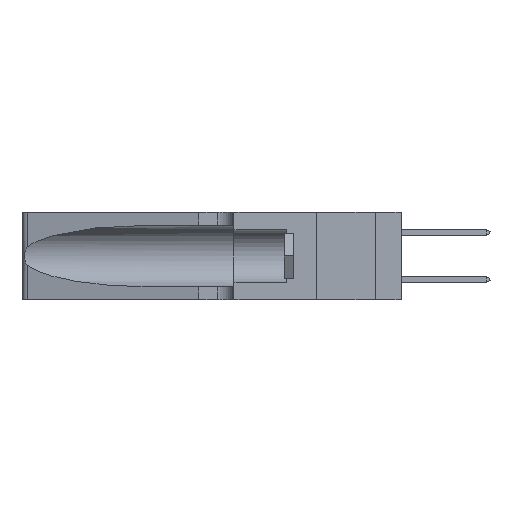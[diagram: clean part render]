
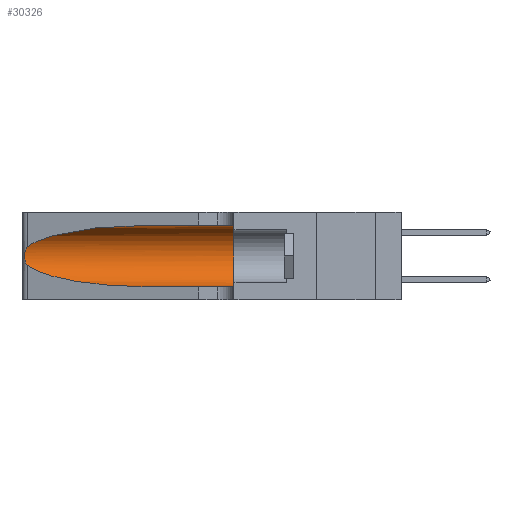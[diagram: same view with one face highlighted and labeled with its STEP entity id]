
A CAD part, left-side view. The second image highlights one B-rep face of the part: STEP entity #30326.
In plain terms, the highlighted cylindrical face has radius 3.308 mm (diameter 6.617 mm), a partial arc.
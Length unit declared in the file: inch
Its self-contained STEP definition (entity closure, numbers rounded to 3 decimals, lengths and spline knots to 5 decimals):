
#28 = ORIENTED_EDGE ( 'NONE', *, *, #17011, .T. ) ;
#201 = CARTESIAN_POINT ( 'NONE',  ( 0.25487, 1.22718, 0.22369 ) ) ;
#350 = CARTESIAN_POINT ( 'NONE',  ( 0.25639, 1.23186, 0.15144 ) ) ;
#483 = VECTOR ( 'NONE', #36586, 39.37008 ) ;
#2564 = AXIS2_PLACEMENT_3D ( 'NONE', #32352, #11757, #35770 ) ;
#2771 = CARTESIAN_POINT ( 'NONE',  ( 0.18966, 0.96281, 0.31525 ) ) ;
#3012 = CARTESIAN_POINT ( 'NONE',  ( 0.1305, 0.35, 0.31525 ) ) ;
#3841 = CARTESIAN_POINT ( 'NONE',  ( 0.25487, 1.22718, 0.14631 ) ) ;
#4213 = CARTESIAN_POINT ( 'NONE',  ( 0.2373, 1.15595, 0.08982 ) ) ;
#4339 = CARTESIAN_POINT ( 'NONE',  ( 0.1305, 0.35, 0.05475 ) ) ;
#5648 = CARTESIAN_POINT ( 'NONE',  ( 0.1305, 1.61858, 0.31525 ) ) ;
#6294 = CARTESIAN_POINT ( 'NONE',  ( 0.2373, 1.15595, 0.28018 ) ) ;
#7116 = VERTEX_POINT ( 'NONE', #38275 ) ;
#7188 = CARTESIAN_POINT ( 'NONE',  ( 0.25639, 1.23184, 0.21858 ) ) ;
#8153 = ORIENTED_EDGE ( 'NONE', *, *, #41227, .T. ) ;
#9260 = DIRECTION ( 'NONE',  ( 0., 0., -1. ) ) ;
#9715 = LINE ( 'NONE', #5648, #483 ) ;
#10643 = CARTESIAN_POINT ( 'NONE',  ( 0.25854, 1.2359, 0.20912 ) ) ;
#11147 = CARTESIAN_POINT ( 'NONE',  ( 0.1305, 0.72297, 0.05475 ) ) ;
#11757 = DIRECTION ( 'NONE',  ( 0., 1., 0. ) ) ;
#12356 = VERTEX_POINT ( 'NONE', #4339 ) ;
#14110 = CARTESIAN_POINT ( 'NONE',  ( 0.26075, 1.23896, 0.19203 ) ) ;
#14637 = ORIENTED_EDGE ( 'NONE', *, *, #16040, .F. ) ;
#16040 = EDGE_CURVE ( 'NONE', #32694, #33945, #9715, .T. ) ;
#16233 = VECTOR ( 'NONE', #33271, 39.37008 ) ;
#16890 = CIRCLE ( 'NONE', #2564, 0.13025 ) ;
#17011 = EDGE_CURVE ( 'NONE', #7116, #24454, #36749, .T. ) ;
#17569 = CARTESIAN_POINT ( 'NONE',  ( 0.26017, 1.23833, 0.17102 ) ) ;
#18398 = ORIENTED_EDGE ( 'NONE', *, *, #20824, .T. ) ;
#20617 = CYLINDRICAL_SURFACE ( 'NONE', #24099, 0.13025 ) ;
#20822 =( BOUNDED_CURVE ( )  B_SPLINE_CURVE ( 3, ( #28304, #4213, #31745, #11147 ),
 .UNSPECIFIED., .F., .F. ) 
 B_SPLINE_CURVE_WITH_KNOTS ( ( 4, 4 ),
 ( 3.44316, 4.71239 ),
 .UNSPECIFIED. ) 
 CURVE ( )  GEOMETRIC_REPRESENTATION_ITEM ( )  RATIONAL_B_SPLINE_CURVE ( ( 1., 0.87, 0.87, 1. ) ) 
 REPRESENTATION_ITEM ( '' )  );
#20824 = EDGE_CURVE ( 'NONE', #24454, #41369, #20822, .T. ) ;
#20894 = CARTESIAN_POINT ( 'NONE',  ( 0.25555, 1.22994, 0.2215 ) ) ;
#21042 = CARTESIAN_POINT ( 'NONE',  ( 0.25789, 1.23486, 0.15765 ) ) ;
#21650 = ORIENTED_EDGE ( 'NONE', *, *, #35269, .F. ) ;
#22866 = CARTESIAN_POINT ( 'NONE',  ( 0.25487, 1.22718, 0.14631 ) ) ;
#22958 = CARTESIAN_POINT ( 'NONE',  ( 0.1305, 1.61858, 0.185 ) ) ;
#24099 = AXIS2_PLACEMENT_3D ( 'NONE', #22958, #29871, #9260 ) ;
#24454 = VERTEX_POINT ( 'NONE', #22866 ) ;
#24498 = CARTESIAN_POINT ( 'NONE',  ( 0.25555, 1.22993, 0.14849 ) ) ;
#25496 =( BOUNDED_CURVE ( )  B_SPLINE_CURVE ( 3, ( #26918, #2771, #6294, #30357 ),
 .UNSPECIFIED., .F., .T. ) 
 B_SPLINE_CURVE_WITH_KNOTS ( ( 4, 4 ),
 ( 1.5708, 2.84003 ),
 .UNSPECIFIED. ) 
 CURVE ( )  GEOMETRIC_REPRESENTATION_ITEM ( )  RATIONAL_B_SPLINE_CURVE ( ( 1., 0.87, 0.87, 1. ) ) 
 REPRESENTATION_ITEM ( '' )  );
#25670 = EDGE_LOOP ( 'NONE', ( #8153, #28, #18398, #29700, #21650, #14637 ) ) ;
#26918 = CARTESIAN_POINT ( 'NONE',  ( 0.1305, 0.72297, 0.31525 ) ) ;
#28304 = CARTESIAN_POINT ( 'NONE',  ( 0.25487, 1.22718, 0.14631 ) ) ;
#29700 = ORIENTED_EDGE ( 'NONE', *, *, #30838, .T. ) ;
#29840 = CARTESIAN_POINT ( 'NONE',  ( 0.1305, 1.61858, 0.05475 ) ) ;
#29871 = DIRECTION ( 'NONE',  ( 0., -1., 0. ) ) ;
#30326 = ADVANCED_FACE ( 'NONE', ( #39856 ), #20617, .F. ) ;
#30357 = CARTESIAN_POINT ( 'NONE',  ( 0.25487, 1.22718, 0.22369 ) ) ;
#30838 = EDGE_CURVE ( 'NONE', #41369, #12356, #35558, .T. ) ;
#31250 = CARTESIAN_POINT ( 'NONE',  ( 0.25787, 1.23484, 0.2124 ) ) ;
#31745 = CARTESIAN_POINT ( 'NONE',  ( 0.18966, 0.96281, 0.05475 ) ) ;
#32352 = CARTESIAN_POINT ( 'NONE',  ( 0.1305, 0.35, 0.185 ) ) ;
#32694 = VERTEX_POINT ( 'NONE', #41236 ) ;
#33271 = DIRECTION ( 'NONE',  ( 0., -1., 0. ) ) ;
#33945 = VERTEX_POINT ( 'NONE', #3012 ) ;
#34655 = CARTESIAN_POINT ( 'NONE',  ( 0.26018, 1.23835, 0.19895 ) ) ;
#35269 = EDGE_CURVE ( 'NONE', #33945, #12356, #16890, .T. ) ;
#35558 = LINE ( 'NONE', #29840, #16233 ) ;
#35770 = DIRECTION ( 'NONE',  ( 0., 0., 1. ) ) ;
#36586 = DIRECTION ( 'NONE',  ( 0., -1., 0. ) ) ;
#36749 = B_SPLINE_CURVE_WITH_KNOTS ( 'NONE', 3,
 ( #201, #20894, #7188, #31250, #10643, #34655, #14110, #38097, #17569, #41493, #21042, #350, #24498, #3841 ),
 .UNSPECIFIED., .F., .F.,
 ( 4, 2, 2, 2, 2, 2, 4 ),
 ( 0., 0.00027, 0.00053, 0.00107, 0.0016, 0.00187, 0.00214 ),
 .UNSPECIFIED. ) ;
#37949 = CARTESIAN_POINT ( 'NONE',  ( 0.1305, 0.72297, 0.05475 ) ) ;
#38097 = CARTESIAN_POINT ( 'NONE',  ( 0.26075, 1.23896, 0.178 ) ) ;
#38275 = CARTESIAN_POINT ( 'NONE',  ( 0.25487, 1.22718, 0.22369 ) ) ;
#39856 = FACE_OUTER_BOUND ( 'NONE', #25670, .T. ) ;
#41227 = EDGE_CURVE ( 'NONE', #32694, #7116, #25496, .T. ) ;
#41236 = CARTESIAN_POINT ( 'NONE',  ( 0.1305, 0.72297, 0.31525 ) ) ;
#41369 = VERTEX_POINT ( 'NONE', #37949 ) ;
#41493 = CARTESIAN_POINT ( 'NONE',  ( 0.25856, 1.23593, 0.16098 ) ) ;
